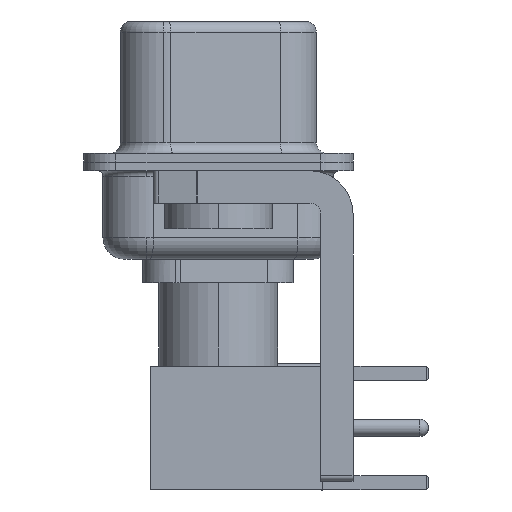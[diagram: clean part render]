
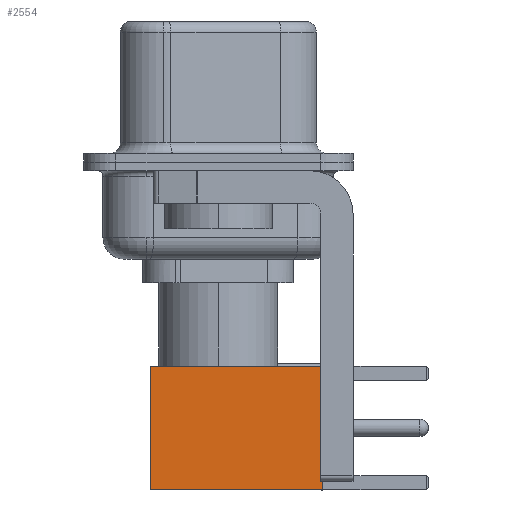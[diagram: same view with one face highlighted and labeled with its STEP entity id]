
A CAD part, left-side view. The second image highlights one B-rep face of the part: STEP entity #2554.
In plain terms, the highlighted face is planar.
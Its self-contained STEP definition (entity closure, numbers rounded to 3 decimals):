
#320 = EDGE_CURVE ( 'NONE', #636, #24657, #2484, .T. ) ;
#636 = VERTEX_POINT ( 'NONE', #14769 ) ;
#908 = CARTESIAN_POINT ( 'NONE',  ( -2.875, 2.875, 8. ) ) ;
#1891 = VERTEX_POINT ( 'NONE', #8555 ) ;
#2484 = LINE ( 'NONE', #8932, #23435 ) ;
#2554 = ADVANCED_FACE ( 'NONE', ( #27196 ), #25054, .T. ) ;
#2912 = DIRECTION ( 'NONE',  ( -1., 0., 0. ) ) ;
#3022 = DIRECTION ( 'NONE',  ( 0., 1., 0. ) ) ;
#3529 = VECTOR ( 'NONE', #12689, 1000. ) ;
#4385 = CARTESIAN_POINT ( 'NONE',  ( -2.875, 2.875, 0. ) ) ;
#4522 = LINE ( 'NONE', #4385, #3529 ) ;
#4712 = DIRECTION ( 'NONE',  ( 0., 0., -1. ) ) ;
#4895 = ORIENTED_EDGE ( 'NONE', *, *, #320, .T. ) ;
#5217 = EDGE_CURVE ( 'NONE', #11892, #24657, #4522, .T. ) ;
#5291 = CARTESIAN_POINT ( 'NONE',  ( 0., 2.875, 8. ) ) ;
#5754 = AXIS2_PLACEMENT_3D ( 'NONE', #11896, #3022, #25197 ) ;
#6266 = ORIENTED_EDGE ( 'NONE', *, *, #5217, .F. ) ;
#8555 = CARTESIAN_POINT ( 'NONE',  ( 2.875, 2.875, 8. ) ) ;
#8932 = CARTESIAN_POINT ( 'NONE',  ( 0., 2.875, 0. ) ) ;
#9715 = DIRECTION ( 'NONE',  ( -1., 0., 0. ) ) ;
#11008 = CARTESIAN_POINT ( 'NONE',  ( 2.875, 2.875, 0. ) ) ;
#11645 = ORIENTED_EDGE ( 'NONE', *, *, #23733, .F. ) ;
#11892 = VERTEX_POINT ( 'NONE', #908 ) ;
#11896 = CARTESIAN_POINT ( 'NONE',  ( 2.875, 2.875, 0. ) ) ;
#12087 = CARTESIAN_POINT ( 'NONE',  ( -2.875, 2.875, 0. ) ) ;
#12294 = LINE ( 'NONE', #5291, #20063 ) ;
#12689 = DIRECTION ( 'NONE',  ( 0., 0., -1. ) ) ;
#14769 = CARTESIAN_POINT ( 'NONE',  ( 2.875, 2.875, 0. ) ) ;
#16661 = EDGE_CURVE ( 'NONE', #1891, #636, #22296, .T. ) ;
#20063 = VECTOR ( 'NONE', #9715, 1000. ) ;
#21027 = ORIENTED_EDGE ( 'NONE', *, *, #16661, .T. ) ;
#21501 = EDGE_LOOP ( 'NONE', ( #21027, #4895, #6266, #11645 ) ) ;
#21619 = VECTOR ( 'NONE', #4712, 1000. ) ;
#22296 = LINE ( 'NONE', #11008, #21619 ) ;
#23435 = VECTOR ( 'NONE', #2912, 1000. ) ;
#23733 = EDGE_CURVE ( 'NONE', #1891, #11892, #12294, .T. ) ;
#24657 = VERTEX_POINT ( 'NONE', #12087 ) ;
#25054 = PLANE ( 'NONE',  #5754 ) ;
#25197 = DIRECTION ( 'NONE',  ( 0., 0., 1. ) ) ;
#27196 = FACE_OUTER_BOUND ( 'NONE', #21501, .T. ) ;
